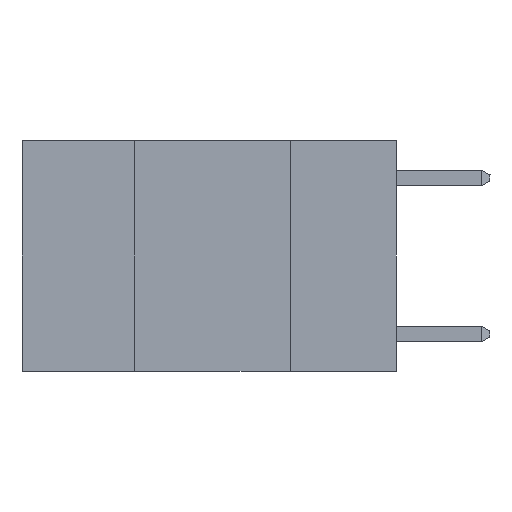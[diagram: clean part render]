
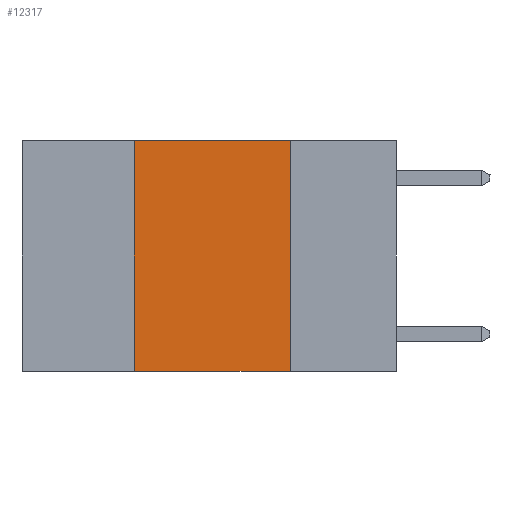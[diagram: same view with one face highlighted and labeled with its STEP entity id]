
A CAD part, left-side view. The second image highlights one B-rep face of the part: STEP entity #12317.
In plain terms, the highlighted planar face has unit normal (-1, 0, 0).
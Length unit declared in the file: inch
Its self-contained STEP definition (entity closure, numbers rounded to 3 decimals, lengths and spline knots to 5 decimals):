
#429 = CARTESIAN_POINT ( 'NONE',  ( 0., 0.17, 0. ) ) ;
#451 = VERTEX_POINT ( 'NONE', #11016 ) ;
#472 = VERTEX_POINT ( 'NONE', #955 ) ;
#733 = LINE ( 'NONE', #13097, #12380 ) ;
#955 = CARTESIAN_POINT ( 'NONE',  ( 0., 0.42, 0. ) ) ;
#2226 = CARTESIAN_POINT ( 'NONE',  ( 0., 0.17, -0.37 ) ) ;
#3902 = ORIENTED_EDGE ( 'NONE', *, *, #10653, .T. ) ;
#4342 = VERTEX_POINT ( 'NONE', #429 ) ;
#5458 = CARTESIAN_POINT ( 'NONE',  ( 0., 0.17, 0. ) ) ;
#5921 = DIRECTION ( 'NONE',  ( 1., 0., 0. ) ) ;
#6169 = DIRECTION ( 'NONE',  ( 0., -1., 0. ) ) ;
#6902 = DIRECTION ( 'NONE',  ( 0., 0., 1. ) ) ;
#7038 = EDGE_CURVE ( 'NONE', #4342, #15948, #7193, .T. ) ;
#7193 = LINE ( 'NONE', #5458, #15203 ) ;
#9384 = DIRECTION ( 'NONE',  ( 0., 0., -1. ) ) ;
#10653 = EDGE_CURVE ( 'NONE', #451, #15948, #733, .T. ) ;
#11016 = CARTESIAN_POINT ( 'NONE',  ( 0., 0.42, -0.37 ) ) ;
#12317 = ADVANCED_FACE ( 'NONE', ( #18249 ), #15013, .F. ) ;
#12380 = VECTOR ( 'NONE', #6169, 39.37008 ) ;
#12527 = CARTESIAN_POINT ( 'NONE',  ( 0., 0.42, 0. ) ) ;
#13097 = CARTESIAN_POINT ( 'NONE',  ( 0., 0.6, -0.37 ) ) ;
#13364 = EDGE_CURVE ( 'NONE', #472, #4342, #20399, .T. ) ;
#13876 = DIRECTION ( 'NONE',  ( 0., 0., -1. ) ) ;
#14650 = AXIS2_PLACEMENT_3D ( 'NONE', #18473, #5921, #9384 ) ;
#15013 = PLANE ( 'NONE',  #14650 ) ;
#15203 = VECTOR ( 'NONE', #13876, 39.37008 ) ;
#15346 = EDGE_CURVE ( 'NONE', #451, #472, #16122, .T. ) ;
#15948 = VERTEX_POINT ( 'NONE', #2226 ) ;
#15987 = ORIENTED_EDGE ( 'NONE', *, *, #7038, .F. ) ;
#16122 = LINE ( 'NONE', #12527, #21347 ) ;
#18249 = FACE_OUTER_BOUND ( 'NONE', #22007, .T. ) ;
#18473 = CARTESIAN_POINT ( 'NONE',  ( 0., 0.6, 0. ) ) ;
#18650 = DIRECTION ( 'NONE',  ( 0., -1., 0. ) ) ;
#19428 = VECTOR ( 'NONE', #18650, 39.37008 ) ;
#20345 = ORIENTED_EDGE ( 'NONE', *, *, #13364, .F. ) ;
#20399 = LINE ( 'NONE', #22486, #19428 ) ;
#21143 = ORIENTED_EDGE ( 'NONE', *, *, #15346, .F. ) ;
#21347 = VECTOR ( 'NONE', #6902, 39.37008 ) ;
#22007 = EDGE_LOOP ( 'NONE', ( #15987, #20345, #21143, #3902 ) ) ;
#22486 = CARTESIAN_POINT ( 'NONE',  ( 0., 0.6, 0. ) ) ;
